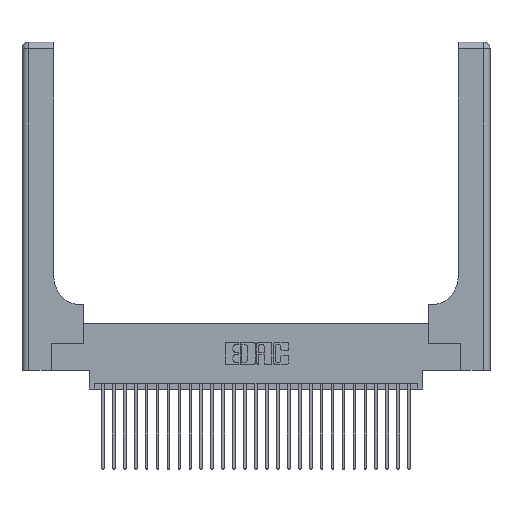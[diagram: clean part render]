
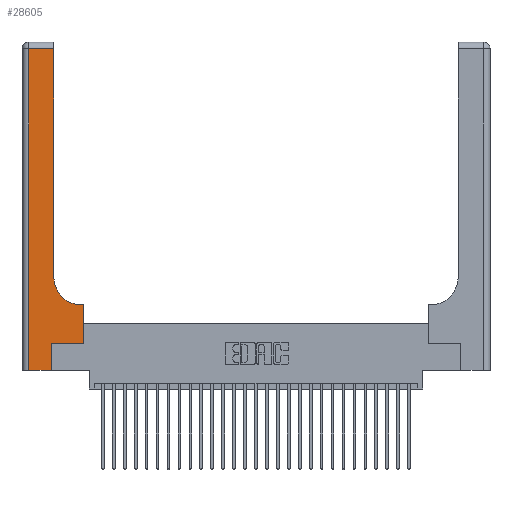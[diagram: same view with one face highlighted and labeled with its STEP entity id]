
A CAD part, top view. The second image highlights one B-rep face of the part: STEP entity #28605.
In plain terms, the highlighted planar face has unit normal (0, 0, 1).
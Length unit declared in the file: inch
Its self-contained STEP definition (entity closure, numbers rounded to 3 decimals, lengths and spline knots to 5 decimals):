
#90 = EDGE_CURVE ( 'NONE', #24734, #8010, #26406, .T. ) ;
#567 = CARTESIAN_POINT ( 'NONE',  ( 0.2915, 0.6, 0.37 ) ) ;
#943 = EDGE_CURVE ( 'NONE', #17260, #24734, #25648, .T. ) ;
#1305 = CARTESIAN_POINT ( 'NONE',  ( 0.5585, 0.6, 0.37 ) ) ;
#1533 = FACE_OUTER_BOUND ( 'NONE', #20225, .T. ) ;
#2166 = ORIENTED_EDGE ( 'NONE', *, *, #6274, .T. ) ;
#2252 = VECTOR ( 'NONE', #14768, 39.37008 ) ;
#2777 = CARTESIAN_POINT ( 'NONE',  ( 0.06, 3., 0.37 ) ) ;
#3187 = VECTOR ( 'NONE', #5203, 39.37008 ) ;
#3574 = VERTEX_POINT ( 'NONE', #6664 ) ;
#3676 = LINE ( 'NONE', #8178, #22469 ) ;
#3794 = VECTOR ( 'NONE', #25676, 39.37008 ) ;
#4609 = DIRECTION ( 'NONE',  ( 0., 1., 0. ) ) ;
#4622 = EDGE_CURVE ( 'NONE', #25836, #10978, #21320, .T. ) ;
#4775 = CARTESIAN_POINT ( 'NONE',  ( 0.5415, 0.85, 0.37 ) ) ;
#5203 = DIRECTION ( 'NONE',  ( -1., 0., 0. ) ) ;
#5231 = DIRECTION ( 'NONE',  ( 1., 0., 0. ) ) ;
#6274 = EDGE_CURVE ( 'NONE', #6884, #3574, #26276, .T. ) ;
#6363 = EDGE_CURVE ( 'NONE', #23900, #6884, #21593, .T. ) ;
#6664 = CARTESIAN_POINT ( 'NONE',  ( 0.2915, 0.85, 0.37 ) ) ;
#6884 = VERTEX_POINT ( 'NONE', #11389 ) ;
#6981 = LINE ( 'NONE', #15192, #11340 ) ;
#7619 = ORIENTED_EDGE ( 'NONE', *, *, #13672, .T. ) ;
#7984 = EDGE_CURVE ( 'NONE', #8010, #20884, #21820, .T. ) ;
#8010 = VERTEX_POINT ( 'NONE', #19377 ) ;
#8178 = CARTESIAN_POINT ( 'NONE',  ( 0.2915, 3., 0.37 ) ) ;
#8188 = DIRECTION ( 'NONE',  ( 0., 1., 0. ) ) ;
#8287 = ORIENTED_EDGE ( 'NONE', *, *, #4622, .T. ) ;
#10348 = DIRECTION ( 'NONE',  ( 0., 0., -1. ) ) ;
#10361 = CARTESIAN_POINT ( 'NONE',  ( 0.2915, 2.94, 0.37 ) ) ;
#10978 = VERTEX_POINT ( 'NONE', #13254 ) ;
#11076 = DIRECTION ( 'NONE',  ( 0., 1., 0. ) ) ;
#11340 = VECTOR ( 'NONE', #8188, 39.37008 ) ;
#11389 = CARTESIAN_POINT ( 'NONE',  ( 0.5415, 0.6, 0.37 ) ) ;
#12709 = VECTOR ( 'NONE', #5231, 39.37008 ) ;
#12886 = CARTESIAN_POINT ( 'NONE',  ( 0., 2.94, 0.37 ) ) ;
#13035 = VECTOR ( 'NONE', #11076, 39.37008 ) ;
#13254 = CARTESIAN_POINT ( 'NONE',  ( 0.5585, 0.25, 0.37 ) ) ;
#13672 = EDGE_CURVE ( 'NONE', #10978, #23900, #13746, .T. ) ;
#13746 = LINE ( 'NONE', #24869, #13035 ) ;
#14114 = VECTOR ( 'NONE', #24750, 39.37008 ) ;
#14386 = CARTESIAN_POINT ( 'NONE',  ( 0.269, 0.25, 0.37 ) ) ;
#14768 = DIRECTION ( 'NONE',  ( 0., -1., 0. ) ) ;
#14820 = AXIS2_PLACEMENT_3D ( 'NONE', #15054, #10348, #15246 ) ;
#15054 = CARTESIAN_POINT ( 'NONE',  ( 0., 3., 0.37 ) ) ;
#15192 = CARTESIAN_POINT ( 'NONE',  ( 0.269, 0., 0.37 ) ) ;
#15246 = DIRECTION ( 'NONE',  ( -1., 0., 0. ) ) ;
#15303 = ORIENTED_EDGE ( 'NONE', *, *, #90, .T. ) ;
#16587 = CARTESIAN_POINT ( 'NONE',  ( 0.06, 2.94, 0.37 ) ) ;
#16993 = EDGE_CURVE ( 'NONE', #20884, #25836, #6981, .T. ) ;
#17260 = VERTEX_POINT ( 'NONE', #10361 ) ;
#17625 = EDGE_CURVE ( 'NONE', #3574, #17260, #3676, .T. ) ;
#18585 = ORIENTED_EDGE ( 'NONE', *, *, #943, .T. ) ;
#19377 = CARTESIAN_POINT ( 'NONE',  ( 0.06, 0., 0.37 ) ) ;
#20225 = EDGE_LOOP ( 'NONE', ( #24695, #18585, #15303, #29284, #25583, #8287, #7619, #28715, #2166 ) ) ;
#20884 = VERTEX_POINT ( 'NONE', #21667 ) ;
#21095 = DIRECTION ( 'NONE',  ( 1., 0., 0. ) ) ;
#21320 = LINE ( 'NONE', #14386, #12709 ) ;
#21593 = LINE ( 'NONE', #567, #3187 ) ;
#21667 = CARTESIAN_POINT ( 'NONE',  ( 0.269, 0., 0.37 ) ) ;
#21820 = LINE ( 'NONE', #26075, #3794 ) ;
#21824 = PLANE ( 'NONE',  #14820 ) ;
#22469 = VECTOR ( 'NONE', #4609, 39.37008 ) ;
#23900 = VERTEX_POINT ( 'NONE', #1305 ) ;
#24695 = ORIENTED_EDGE ( 'NONE', *, *, #17625, .T. ) ;
#24734 = VERTEX_POINT ( 'NONE', #16587 ) ;
#24750 = DIRECTION ( 'NONE',  ( -1., 0., 0. ) ) ;
#24869 = CARTESIAN_POINT ( 'NONE',  ( 0.5585, 0.25, 0.37 ) ) ;
#25583 = ORIENTED_EDGE ( 'NONE', *, *, #16993, .T. ) ;
#25627 = DIRECTION ( 'NONE',  ( 0., 0., -1. ) ) ;
#25648 = LINE ( 'NONE', #12886, #14114 ) ;
#25676 = DIRECTION ( 'NONE',  ( 1., 0., 0. ) ) ;
#25836 = VERTEX_POINT ( 'NONE', #29559 ) ;
#26075 = CARTESIAN_POINT ( 'NONE',  ( 0., 0., 0.37 ) ) ;
#26276 = CIRCLE ( 'NONE', #26623, 0.25 ) ;
#26406 = LINE ( 'NONE', #2777, #2252 ) ;
#26623 = AXIS2_PLACEMENT_3D ( 'NONE', #4775, #25627, #21095 ) ;
#28605 = ADVANCED_FACE ( 'NONE', ( #1533 ), #21824, .F. ) ;
#28715 = ORIENTED_EDGE ( 'NONE', *, *, #6363, .T. ) ;
#29284 = ORIENTED_EDGE ( 'NONE', *, *, #7984, .T. ) ;
#29559 = CARTESIAN_POINT ( 'NONE',  ( 0.269, 0.25, 0.37 ) ) ;
